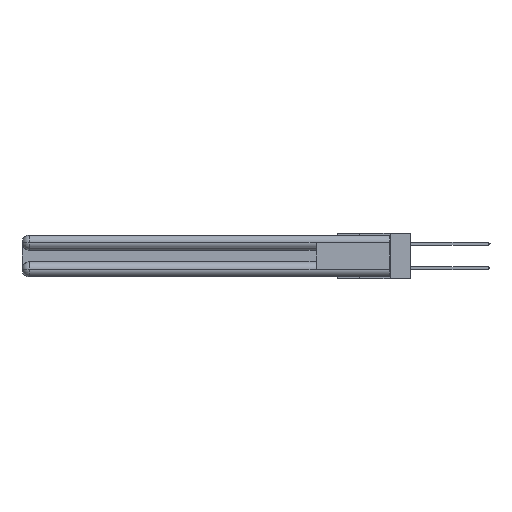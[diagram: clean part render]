
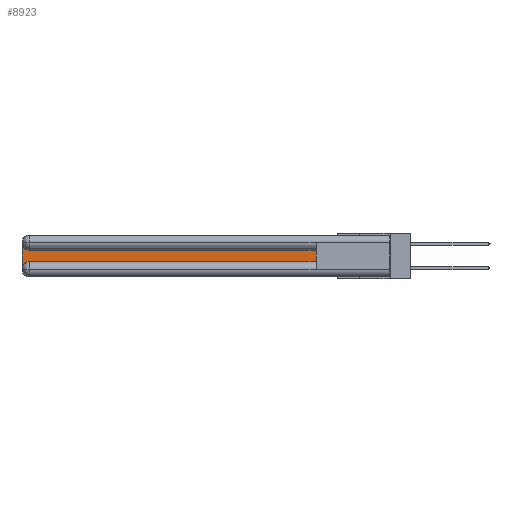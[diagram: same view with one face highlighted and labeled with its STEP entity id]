
A CAD part, left-side view. The second image highlights one B-rep face of the part: STEP entity #8923.
In plain terms, the highlighted planar face has unit normal (-1, 0, 0).
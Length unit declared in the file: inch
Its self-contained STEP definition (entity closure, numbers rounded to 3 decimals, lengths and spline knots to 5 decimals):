
#169 = CARTESIAN_POINT ( 'NONE',  ( 0.075, 0.6, -0.1225 ) ) ;
#995 = PLANE ( 'NONE',  #6974 ) ;
#2373 = EDGE_CURVE ( 'NONE', #26335, #19193, #5975, .T. ) ;
#3094 = CARTESIAN_POINT ( 'NONE',  ( 0.075, 2.94, -0.2775 ) ) ;
#3398 = CARTESIAN_POINT ( 'NONE',  ( 0.075, 3., -0.2175 ) ) ;
#4225 = CIRCLE ( 'NONE', #11183, 0.06 ) ;
#5042 = DIRECTION ( 'NONE',  ( 1., 0., 0. ) ) ;
#5084 = DIRECTION ( 'NONE',  ( 1., 0., 0. ) ) ;
#5147 = EDGE_CURVE ( 'NONE', #26518, #21488, #22541, .T. ) ;
#5401 = DIRECTION ( 'NONE',  ( 0., 0., -1. ) ) ;
#5683 = CARTESIAN_POINT ( 'NONE',  ( 0.075, 0.6, -0.2175 ) ) ;
#5742 = CARTESIAN_POINT ( 'NONE',  ( 0.075, 2.94, -0.1225 ) ) ;
#5975 = LINE ( 'NONE', #3398, #6317 ) ;
#6317 = VECTOR ( 'NONE', #23193, 39.37008 ) ;
#6810 = DIRECTION ( 'NONE',  ( 0., 1., 0. ) ) ;
#6974 = AXIS2_PLACEMENT_3D ( 'NONE', #12574, #21738, #12489 ) ;
#8003 = VERTEX_POINT ( 'NONE', #5742 ) ;
#8277 = EDGE_CURVE ( 'NONE', #17915, #26518, #23322, .T. ) ;
#8880 = EDGE_CURVE ( 'NONE', #19193, #17915, #10814, .T. ) ;
#8923 = ADVANCED_FACE ( 'NONE', ( #22218 ), #995, .F. ) ;
#9102 = DIRECTION ( 'NONE',  ( 0., -1., 0. ) ) ;
#10814 = CIRCLE ( 'NONE', #10982, 0.06 ) ;
#10982 = AXIS2_PLACEMENT_3D ( 'NONE', #3094, #5084, #5401 ) ;
#11160 = EDGE_CURVE ( 'NONE', #8003, #26335, #4225, .T. ) ;
#11183 = AXIS2_PLACEMENT_3D ( 'NONE', #25470, #5042, #16596 ) ;
#11471 = ORIENTED_EDGE ( 'NONE', *, *, #5147, .T. ) ;
#11760 = EDGE_LOOP ( 'NONE', ( #29070, #17212, #17764, #23102, #18564, #11471 ) ) ;
#11868 = VECTOR ( 'NONE', #23898, 39.37008 ) ;
#12255 = LINE ( 'NONE', #169, #22911 ) ;
#12489 = DIRECTION ( 'NONE',  ( 0., 0., -1. ) ) ;
#12574 = CARTESIAN_POINT ( 'NONE',  ( 0.075, 3., -0.1225 ) ) ;
#14649 = CARTESIAN_POINT ( 'NONE',  ( 0.075, 2.94, -0.2175 ) ) ;
#16596 = DIRECTION ( 'NONE',  ( 0., 0., -1. ) ) ;
#17212 = ORIENTED_EDGE ( 'NONE', *, *, #11160, .T. ) ;
#17764 = ORIENTED_EDGE ( 'NONE', *, *, #2373, .T. ) ;
#17915 = VERTEX_POINT ( 'NONE', #14649 ) ;
#18564 = ORIENTED_EDGE ( 'NONE', *, *, #8277, .T. ) ;
#19193 = VERTEX_POINT ( 'NONE', #21344 ) ;
#21065 = CARTESIAN_POINT ( 'NONE',  ( 0.075, 0.6, -0.1225 ) ) ;
#21344 = CARTESIAN_POINT ( 'NONE',  ( 0.075, 3., -0.2775 ) ) ;
#21488 = VERTEX_POINT ( 'NONE', #21065 ) ;
#21738 = DIRECTION ( 'NONE',  ( 1., 0., 0. ) ) ;
#22218 = FACE_OUTER_BOUND ( 'NONE', #11760, .T. ) ;
#22541 = LINE ( 'NONE', #5683, #11868 ) ;
#22911 = VECTOR ( 'NONE', #6810, 39.37008 ) ;
#23102 = ORIENTED_EDGE ( 'NONE', *, *, #8880, .T. ) ;
#23193 = DIRECTION ( 'NONE',  ( 0., 0., -1. ) ) ;
#23322 = LINE ( 'NONE', #27224, #25823 ) ;
#23898 = DIRECTION ( 'NONE',  ( 0., 0., 1. ) ) ;
#24282 = CARTESIAN_POINT ( 'NONE',  ( 0.075, 3., -0.0625 ) ) ;
#25470 = CARTESIAN_POINT ( 'NONE',  ( 0.075, 2.94, -0.0625 ) ) ;
#25517 = EDGE_CURVE ( 'NONE', #21488, #8003, #12255, .T. ) ;
#25823 = VECTOR ( 'NONE', #9102, 39.37008 ) ;
#26335 = VERTEX_POINT ( 'NONE', #24282 ) ;
#26518 = VERTEX_POINT ( 'NONE', #28109 ) ;
#27224 = CARTESIAN_POINT ( 'NONE',  ( 0.075, 0.6, -0.2175 ) ) ;
#28109 = CARTESIAN_POINT ( 'NONE',  ( 0.075, 0.6, -0.2175 ) ) ;
#29070 = ORIENTED_EDGE ( 'NONE', *, *, #25517, .T. ) ;
